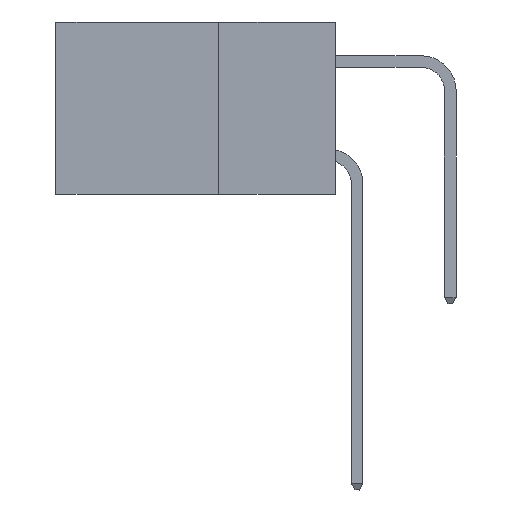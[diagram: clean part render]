
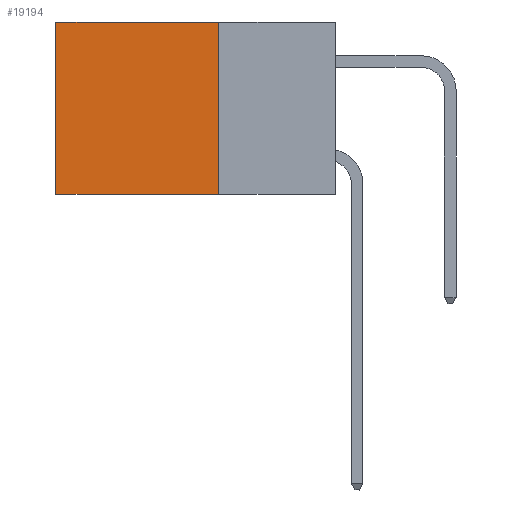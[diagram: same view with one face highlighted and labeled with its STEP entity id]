
A CAD part, left-side view. The second image highlights one B-rep face of the part: STEP entity #19194.
In plain terms, the highlighted planar face has unit normal (-1, 0, 0).
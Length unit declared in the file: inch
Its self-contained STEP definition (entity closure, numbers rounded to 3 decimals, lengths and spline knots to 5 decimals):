
#154 = LINE ( 'NONE', #8593, #22874 ) ;
#398 = CARTESIAN_POINT ( 'NONE',  ( 0.2875, 0.25, -0.37 ) ) ;
#604 = VERTEX_POINT ( 'NONE', #21032 ) ;
#979 = EDGE_CURVE ( 'NONE', #9333, #604, #154, .T. ) ;
#1691 = CARTESIAN_POINT ( 'NONE',  ( 0.2875, 0.25, 0. ) ) ;
#3319 = VERTEX_POINT ( 'NONE', #1691 ) ;
#3591 = AXIS2_PLACEMENT_3D ( 'NONE', #7619, #7198, #15622 ) ;
#4878 = DIRECTION ( 'NONE',  ( 0., 1., 0. ) ) ;
#6270 = EDGE_LOOP ( 'NONE', ( #6439, #11660, #16654, #18920 ) ) ;
#6345 = DIRECTION ( 'NONE',  ( 0., 0., -1. ) ) ;
#6439 = ORIENTED_EDGE ( 'NONE', *, *, #979, .T. ) ;
#6601 = CARTESIAN_POINT ( 'NONE',  ( 0.2875, 0.25, 0. ) ) ;
#7198 = DIRECTION ( 'NONE',  ( 1., 0., 0. ) ) ;
#7411 = VERTEX_POINT ( 'NONE', #398 ) ;
#7619 = CARTESIAN_POINT ( 'NONE',  ( 0.2875, 0.25, 0. ) ) ;
#8556 = VECTOR ( 'NONE', #13110, 39.37008 ) ;
#8593 = CARTESIAN_POINT ( 'NONE',  ( 0.2875, 0.6, 0. ) ) ;
#9325 = CARTESIAN_POINT ( 'NONE',  ( 0.2875, 0.6, 0. ) ) ;
#9333 = VERTEX_POINT ( 'NONE', #9325 ) ;
#11660 = ORIENTED_EDGE ( 'NONE', *, *, #13833, .F. ) ;
#13110 = DIRECTION ( 'NONE',  ( 0., 0., -1. ) ) ;
#13833 = EDGE_CURVE ( 'NONE', #7411, #604, #23987, .T. ) ;
#14205 = VECTOR ( 'NONE', #22172, 39.37008 ) ;
#15622 = DIRECTION ( 'NONE',  ( 0., 0., -1. ) ) ;
#16497 = LINE ( 'NONE', #24917, #25197 ) ;
#16654 = ORIENTED_EDGE ( 'NONE', *, *, #23124, .F. ) ;
#17705 = PLANE ( 'NONE',  #3591 ) ;
#18538 = EDGE_CURVE ( 'NONE', #3319, #9333, #16497, .T. ) ;
#18920 = ORIENTED_EDGE ( 'NONE', *, *, #18538, .T. ) ;
#19194 = ADVANCED_FACE ( 'NONE', ( #19762 ), #17705, .F. ) ;
#19762 = FACE_OUTER_BOUND ( 'NONE', #6270, .T. ) ;
#21032 = CARTESIAN_POINT ( 'NONE',  ( 0.2875, 0.6, -0.37 ) ) ;
#21775 = CARTESIAN_POINT ( 'NONE',  ( 0.2875, 0.25, -0.37 ) ) ;
#22172 = DIRECTION ( 'NONE',  ( 0., 1., 0. ) ) ;
#22874 = VECTOR ( 'NONE', #6345, 39.37008 ) ;
#23124 = EDGE_CURVE ( 'NONE', #3319, #7411, #25524, .T. ) ;
#23987 = LINE ( 'NONE', #21775, #14205 ) ;
#24917 = CARTESIAN_POINT ( 'NONE',  ( 0.2875, 0.25, 0. ) ) ;
#25197 = VECTOR ( 'NONE', #4878, 39.37008 ) ;
#25524 = LINE ( 'NONE', #6601, #8556 ) ;
